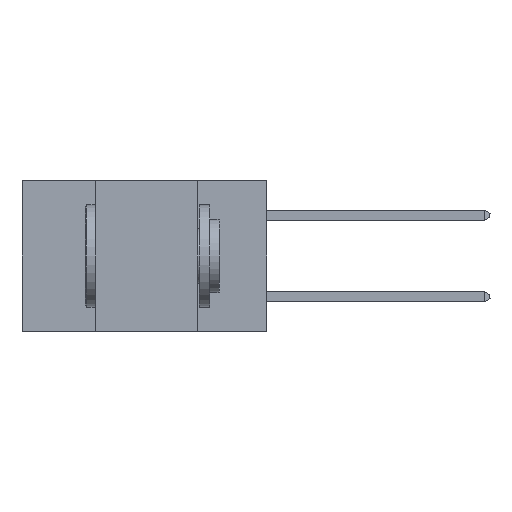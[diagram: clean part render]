
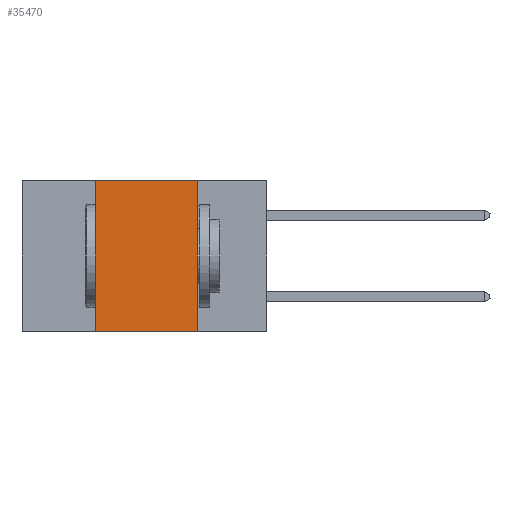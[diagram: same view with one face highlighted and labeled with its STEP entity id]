
A CAD part, left-side view. The second image highlights one B-rep face of the part: STEP entity #35470.
In plain terms, the highlighted planar face has unit normal (-1, 0, 0).
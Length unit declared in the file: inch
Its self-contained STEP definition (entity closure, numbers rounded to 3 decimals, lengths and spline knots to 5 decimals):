
#122 = ORIENTED_EDGE ( 'NONE', *, *, #6198, .F. ) ;
#1222 = EDGE_CURVE ( 'NONE', #9449, #17395, #12715, .T. ) ;
#2609 = CARTESIAN_POINT ( 'NONE',  ( 0., 0.17, 0. ) ) ;
#3830 = VECTOR ( 'NONE', #25905, 39.37008 ) ;
#3993 = CARTESIAN_POINT ( 'NONE',  ( 0., 0.17, 0. ) ) ;
#4275 = AXIS2_PLACEMENT_3D ( 'NONE', #34686, #26593, #10058 ) ;
#5247 = VERTEX_POINT ( 'NONE', #2609 ) ;
#5805 = VECTOR ( 'NONE', #22764, 39.37008 ) ;
#6198 = EDGE_CURVE ( 'NONE', #5247, #17395, #22504, .T. ) ;
#8310 = CARTESIAN_POINT ( 'NONE',  ( 0., 0.17, -0.37 ) ) ;
#9449 = VERTEX_POINT ( 'NONE', #15531 ) ;
#10058 = DIRECTION ( 'NONE',  ( 0., 0., -1. ) ) ;
#10141 = ORIENTED_EDGE ( 'NONE', *, *, #16250, .F. ) ;
#11355 = EDGE_LOOP ( 'NONE', ( #122, #10141, #25701, #33802 ) ) ;
#12142 = DIRECTION ( 'NONE',  ( 0., -1., 0. ) ) ;
#12361 = LINE ( 'NONE', #19989, #5805 ) ;
#12414 = EDGE_CURVE ( 'NONE', #9449, #20850, #12361, .T. ) ;
#12416 = DIRECTION ( 'NONE',  ( 0., 0., -1. ) ) ;
#12715 = LINE ( 'NONE', #34100, #19190 ) ;
#14856 = CARTESIAN_POINT ( 'NONE',  ( 0., 0.6, 0. ) ) ;
#15531 = CARTESIAN_POINT ( 'NONE',  ( 0., 0.42, -0.37 ) ) ;
#16250 = EDGE_CURVE ( 'NONE', #20850, #5247, #25926, .T. ) ;
#17395 = VERTEX_POINT ( 'NONE', #8310 ) ;
#19190 = VECTOR ( 'NONE', #12142, 39.37008 ) ;
#19989 = CARTESIAN_POINT ( 'NONE',  ( 0., 0.42, 0. ) ) ;
#20850 = VERTEX_POINT ( 'NONE', #34949 ) ;
#22504 = LINE ( 'NONE', #3993, #28985 ) ;
#22764 = DIRECTION ( 'NONE',  ( 0., 0., 1. ) ) ;
#23822 = PLANE ( 'NONE',  #4275 ) ;
#25701 = ORIENTED_EDGE ( 'NONE', *, *, #12414, .F. ) ;
#25905 = DIRECTION ( 'NONE',  ( 0., -1., 0. ) ) ;
#25926 = LINE ( 'NONE', #14856, #3830 ) ;
#26593 = DIRECTION ( 'NONE',  ( 1., 0., 0. ) ) ;
#28985 = VECTOR ( 'NONE', #12416, 39.37008 ) ;
#29281 = FACE_OUTER_BOUND ( 'NONE', #11355, .T. ) ;
#33802 = ORIENTED_EDGE ( 'NONE', *, *, #1222, .T. ) ;
#34100 = CARTESIAN_POINT ( 'NONE',  ( 0., 0.6, -0.37 ) ) ;
#34686 = CARTESIAN_POINT ( 'NONE',  ( 0., 0.6, 0. ) ) ;
#34949 = CARTESIAN_POINT ( 'NONE',  ( 0., 0.42, 0. ) ) ;
#35470 = ADVANCED_FACE ( 'NONE', ( #29281 ), #23822, .F. ) ;
